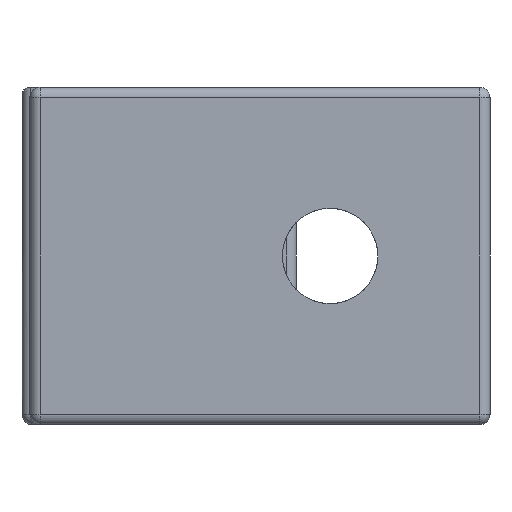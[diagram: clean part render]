
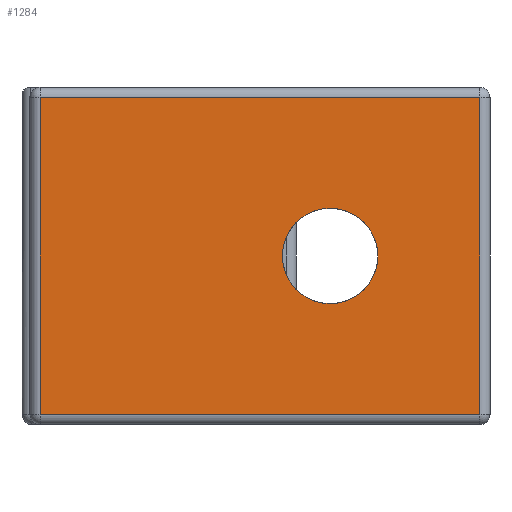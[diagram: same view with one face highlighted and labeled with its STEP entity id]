
A CAD part, front view. The second image highlights one B-rep face of the part: STEP entity #1284.
In plain terms, the highlighted planar face has unit normal (0, -1, 0).
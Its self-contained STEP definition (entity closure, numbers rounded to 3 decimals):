
#15=FACE_BOUND('',#429,.T.);
#29=PLANE('',#1477);
#106=LINE('',#2335,#184);
#111=LINE('',#2409,#189);
#114=LINE('',#2422,#192);
#115=LINE('',#2424,#193);
#184=VECTOR('',#1675,10.);
#189=VECTOR('',#1778,10.);
#192=VECTOR('',#1797,10.);
#193=VECTOR('',#1800,10.);
#340=FACE_OUTER_BOUND('',#428,.T.);
#428=EDGE_LOOP('',(#1170,#1171,#1172,#1173));
#429=EDGE_LOOP('',(#1174));
#539=CIRCLE('',#1478,1.4);
#605=VERTEX_POINT('',#2333);
#606=VERTEX_POINT('',#2334);
#622=VERTEX_POINT('',#2393);
#626=VERTEX_POINT('',#2405);
#638=VERTEX_POINT('',#2524);
#737=EDGE_CURVE('',#605,#606,#106,.T.);
#775=EDGE_CURVE('',#622,#626,#111,.T.);
#782=EDGE_CURVE('',#626,#605,#114,.T.);
#783=EDGE_CURVE('',#606,#622,#115,.T.);
#822=EDGE_CURVE('',#638,#638,#539,.F.);
#1170=ORIENTED_EDGE('',*,*,#775,.F.);
#1171=ORIENTED_EDGE('',*,*,#783,.F.);
#1172=ORIENTED_EDGE('',*,*,#737,.F.);
#1173=ORIENTED_EDGE('',*,*,#782,.F.);
#1174=ORIENTED_EDGE('',*,*,#822,.T.);
#1284=ADVANCED_FACE('',(#340,#15),#29,.F.);
#1477=AXIS2_PLACEMENT_3D('',#2523,#1908,#1909);
#1478=AXIS2_PLACEMENT_3D('',#2525,#1910,#1911);
#1675=DIRECTION('',(1.,0.,0.));
#1778=DIRECTION('',(-1.,0.,0.));
#1797=DIRECTION('',(0.,0.,1.));
#1800=DIRECTION('',(0.,0.,-1.));
#1908=DIRECTION('center_axis',(0.,1.,0.));
#1909=DIRECTION('ref_axis',(1.,0.,0.));
#1910=DIRECTION('center_axis',(0.,-1.,0.));
#1911=DIRECTION('ref_axis',(1.,0.,0.));
#2333=CARTESIAN_POINT('',(0.3,-11.028,10.678));
#2334=CARTESIAN_POINT('',(13.2,-11.028,10.678));
#2335=CARTESIAN_POINT('',(0.345,-11.028,10.678));
#2393=CARTESIAN_POINT('',(13.2,-11.028,1.378));
#2405=CARTESIAN_POINT('',(0.3,-11.028,1.378));
#2409=CARTESIAN_POINT('',(0.,-11.028,1.378));
#2422=CARTESIAN_POINT('',(0.3,-11.028,6.028));
#2424=CARTESIAN_POINT('',(13.2,-11.028,1.028));
#2523=CARTESIAN_POINT('Origin',(0.,-11.028,1.028));
#2524=CARTESIAN_POINT('',(7.409,-11.028,6.028));
#2525=CARTESIAN_POINT('Origin',(8.809,-11.028,6.028));
